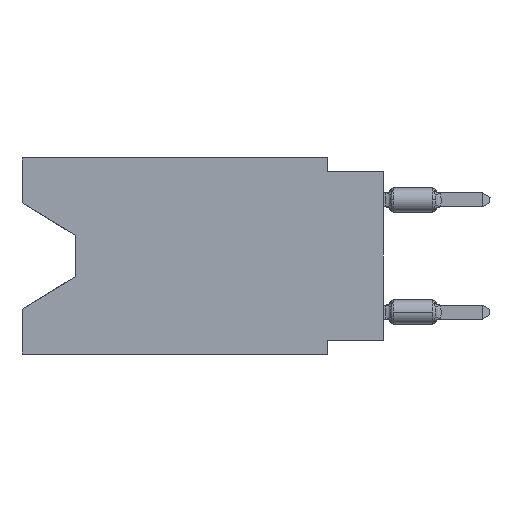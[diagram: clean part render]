
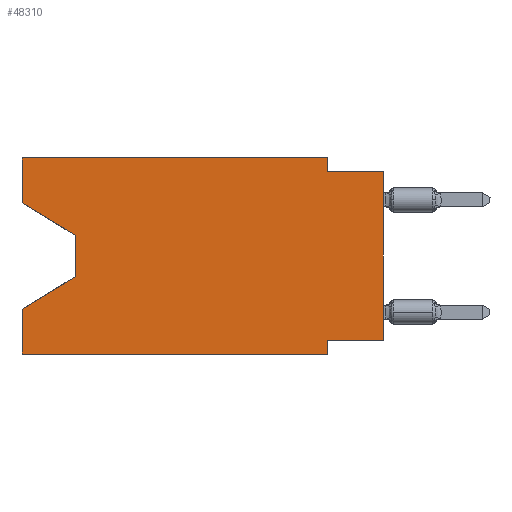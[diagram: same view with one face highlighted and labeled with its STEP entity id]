
A CAD part, left-side view. The second image highlights one B-rep face of the part: STEP entity #48310.
In plain terms, the highlighted planar face has unit normal (-1, 0, 0).
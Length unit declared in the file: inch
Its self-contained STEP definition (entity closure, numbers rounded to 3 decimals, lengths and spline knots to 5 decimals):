
#952 = CARTESIAN_POINT ( 'NONE',  ( 0., 0.1, 0. ) ) ;
#1336 = ORIENTED_EDGE ( 'NONE', *, *, #37360, .F. ) ;
#1438 = EDGE_CURVE ( 'NONE', #51603, #38391, #29458, .T. ) ;
#1773 = LINE ( 'NONE', #55006, #17357 ) ;
#2126 = ORIENTED_EDGE ( 'NONE', *, *, #54145, .F. ) ;
#2921 = DIRECTION ( 'NONE',  ( 0., 0., 1. ) ) ;
#3044 = DIRECTION ( 'NONE',  ( 0., -1., 0. ) ) ;
#4367 = DIRECTION ( 'NONE',  ( 0., 0., -1. ) ) ;
#4669 = VECTOR ( 'NONE', #45339, 39.37008 ) ;
#5023 = VECTOR ( 'NONE', #10471, 39.37008 ) ;
#5188 = LINE ( 'NONE', #31712, #48195 ) ;
#5967 = LINE ( 'NONE', #32765, #39886 ) ;
#6341 = ORIENTED_EDGE ( 'NONE', *, *, #23711, .F. ) ;
#7727 = LINE ( 'NONE', #17108, #21200 ) ;
#8102 = EDGE_LOOP ( 'NONE', ( #10168, #48051, #48409, #39611, #40455, #32962, #37043, #15604, #16162, #6341, #2126, #1336 ) ) ;
#8621 = EDGE_CURVE ( 'NONE', #53166, #44111, #5188, .T. ) ;
#9916 = VECTOR ( 'NONE', #4367, 39.37008 ) ;
#10168 = ORIENTED_EDGE ( 'NONE', *, *, #42761, .T. ) ;
#10471 = DIRECTION ( 'NONE',  ( 0., -0.855, -0.519 ) ) ;
#10531 = DIRECTION ( 'NONE',  ( 0., -1., 0. ) ) ;
#11126 = VECTOR ( 'NONE', #2921, 39.37008 ) ;
#11898 = VERTEX_POINT ( 'NONE', #45254 ) ;
#13742 = VECTOR ( 'NONE', #18275, 39.37008 ) ;
#14012 = CARTESIAN_POINT ( 'NONE',  ( 0., 0.645, 0. ) ) ;
#15604 = ORIENTED_EDGE ( 'NONE', *, *, #38082, .T. ) ;
#16162 = ORIENTED_EDGE ( 'NONE', *, *, #8621, .F. ) ;
#17108 = CARTESIAN_POINT ( 'NONE',  ( 0., 0., 0. ) ) ;
#17289 = CARTESIAN_POINT ( 'NONE',  ( 0., 0.1, 0. ) ) ;
#17357 = VECTOR ( 'NONE', #54439, 39.37008 ) ;
#18275 = DIRECTION ( 'NONE',  ( 0., 0.855, -0.519 ) ) ;
#19020 = CARTESIAN_POINT ( 'NONE',  ( 0., 0.645, 0. ) ) ;
#19334 = CARTESIAN_POINT ( 'NONE',  ( 0., 0.55, -0.138 ) ) ;
#21200 = VECTOR ( 'NONE', #39026, 39.37008 ) ;
#21672 = CARTESIAN_POINT ( 'NONE',  ( 0., 0., -0.025 ) ) ;
#21905 = VECTOR ( 'NONE', #3044, 39.37008 ) ;
#22326 = DIRECTION ( 'NONE',  ( 0., -1., 0. ) ) ;
#23407 = DIRECTION ( 'NONE',  ( 0., 0., -1. ) ) ;
#23504 = CARTESIAN_POINT ( 'NONE',  ( 0., 0.55, -0.212 ) ) ;
#23711 = EDGE_CURVE ( 'NONE', #47330, #53166, #48542, .T. ) ;
#27288 = EDGE_CURVE ( 'NONE', #45841, #51603, #1773, .T. ) ;
#28548 = VECTOR ( 'NONE', #55047, 39.37008 ) ;
#28711 = CARTESIAN_POINT ( 'NONE',  ( 0., 0.645, -0.35 ) ) ;
#28729 = EDGE_CURVE ( 'NONE', #11898, #29575, #51928, .T. ) ;
#29252 = AXIS2_PLACEMENT_3D ( 'NONE', #14012, #48732, #23407 ) ;
#29458 = LINE ( 'NONE', #38527, #28548 ) ;
#29575 = VERTEX_POINT ( 'NONE', #50949 ) ;
#31398 = PLANE ( 'NONE',  #29252 ) ;
#31712 = CARTESIAN_POINT ( 'NONE',  ( 0., 0., -0.025 ) ) ;
#32699 = LINE ( 'NONE', #28711, #21905 ) ;
#32765 = CARTESIAN_POINT ( 'NONE',  ( 0., 0.645, 0. ) ) ;
#32962 = ORIENTED_EDGE ( 'NONE', *, *, #1438, .F. ) ;
#32973 = EDGE_CURVE ( 'NONE', #41320, #29575, #44457, .T. ) ;
#33071 = CARTESIAN_POINT ( 'NONE',  ( 0., 0.1, -0.35 ) ) ;
#33354 = VERTEX_POINT ( 'NONE', #19334 ) ;
#36402 = CARTESIAN_POINT ( 'NONE',  ( 0., 0.645, -0.08025 ) ) ;
#37043 = ORIENTED_EDGE ( 'NONE', *, *, #27288, .F. ) ;
#37360 = EDGE_CURVE ( 'NONE', #39141, #54580, #46489, .T. ) ;
#37700 = CARTESIAN_POINT ( 'NONE',  ( 0., 0., -0.325 ) ) ;
#38082 = EDGE_CURVE ( 'NONE', #45841, #44111, #7727, .T. ) ;
#38391 = VERTEX_POINT ( 'NONE', #33071 ) ;
#38527 = CARTESIAN_POINT ( 'NONE',  ( 0., 0.1, -0.35 ) ) ;
#38818 = DIRECTION ( 'NONE',  ( 0., 0., 1. ) ) ;
#39026 = DIRECTION ( 'NONE',  ( 0., 0., 1. ) ) ;
#39141 = VERTEX_POINT ( 'NONE', #41093 ) ;
#39607 = CARTESIAN_POINT ( 'NONE',  ( 0., 0.55, -0.212 ) ) ;
#39611 = ORIENTED_EDGE ( 'NONE', *, *, #28729, .F. ) ;
#39886 = VECTOR ( 'NONE', #10531, 39.37008 ) ;
#40380 = LINE ( 'NONE', #36402, #5023 ) ;
#40455 = ORIENTED_EDGE ( 'NONE', *, *, #44782, .T. ) ;
#41093 = CARTESIAN_POINT ( 'NONE',  ( 0., 0.645, -0.08025 ) ) ;
#41320 = VERTEX_POINT ( 'NONE', #23504 ) ;
#41928 = CARTESIAN_POINT ( 'NONE',  ( 0., 0.645, 0. ) ) ;
#42761 = EDGE_CURVE ( 'NONE', #39141, #33354, #40380, .T. ) ;
#43131 = EDGE_CURVE ( 'NONE', #33354, #41320, #55271, .T. ) ;
#44111 = VERTEX_POINT ( 'NONE', #21672 ) ;
#44457 = LINE ( 'NONE', #39607, #13742 ) ;
#44782 = EDGE_CURVE ( 'NONE', #11898, #38391, #32699, .T. ) ;
#45254 = CARTESIAN_POINT ( 'NONE',  ( 0., 0.645, -0.35 ) ) ;
#45339 = DIRECTION ( 'NONE',  ( 0., 0., -1. ) ) ;
#45841 = VERTEX_POINT ( 'NONE', #37700 ) ;
#45915 = CARTESIAN_POINT ( 'NONE',  ( 0., 0.55, -0.138 ) ) ;
#46489 = LINE ( 'NONE', #41928, #11126 ) ;
#47330 = VERTEX_POINT ( 'NONE', #17289 ) ;
#48051 = ORIENTED_EDGE ( 'NONE', *, *, #43131, .T. ) ;
#48195 = VECTOR ( 'NONE', #22326, 39.37008 ) ;
#48310 = ADVANCED_FACE ( 'NONE', ( #48472 ), #31398, .F. ) ;
#48409 = ORIENTED_EDGE ( 'NONE', *, *, #32973, .T. ) ;
#48472 = FACE_OUTER_BOUND ( 'NONE', #8102, .T. ) ;
#48542 = LINE ( 'NONE', #952, #9916 ) ;
#48732 = DIRECTION ( 'NONE',  ( 1., 0., 0. ) ) ;
#48998 = CARTESIAN_POINT ( 'NONE',  ( 0., 0.645, 0. ) ) ;
#50195 = VECTOR ( 'NONE', #38818, 39.37008 ) ;
#50949 = CARTESIAN_POINT ( 'NONE',  ( 0., 0.645, -0.26975 ) ) ;
#51603 = VERTEX_POINT ( 'NONE', #54564 ) ;
#51928 = LINE ( 'NONE', #48998, #50195 ) ;
#53103 = CARTESIAN_POINT ( 'NONE',  ( 0., 0.1, -0.025 ) ) ;
#53166 = VERTEX_POINT ( 'NONE', #53103 ) ;
#54145 = EDGE_CURVE ( 'NONE', #54580, #47330, #5967, .T. ) ;
#54439 = DIRECTION ( 'NONE',  ( 0., 1., 0. ) ) ;
#54564 = CARTESIAN_POINT ( 'NONE',  ( 0., 0.1, -0.325 ) ) ;
#54580 = VERTEX_POINT ( 'NONE', #19020 ) ;
#55006 = CARTESIAN_POINT ( 'NONE',  ( 0., 0., -0.325 ) ) ;
#55047 = DIRECTION ( 'NONE',  ( 0., 0., -1. ) ) ;
#55271 = LINE ( 'NONE', #45915, #4669 ) ;
